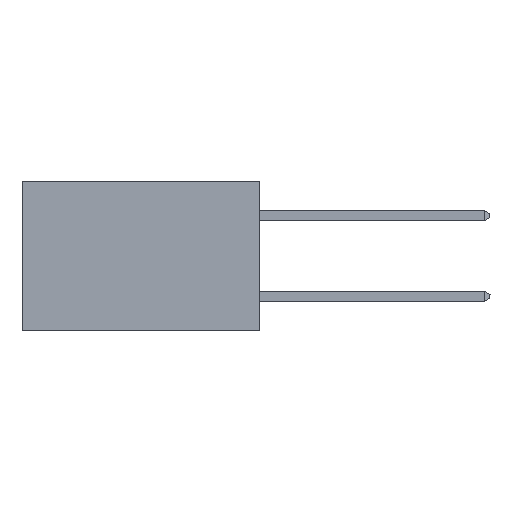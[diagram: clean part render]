
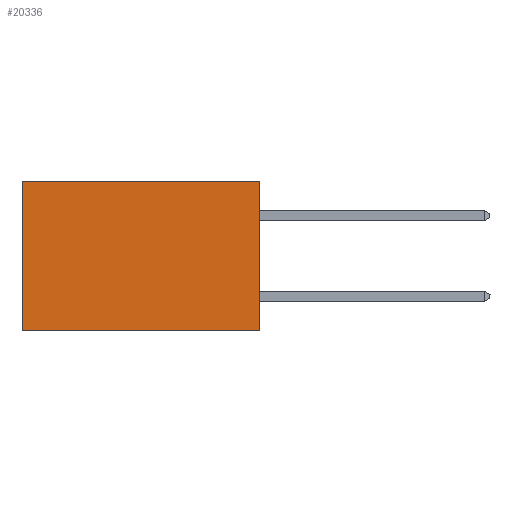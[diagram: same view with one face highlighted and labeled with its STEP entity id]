
A CAD part, left-side view. The second image highlights one B-rep face of the part: STEP entity #20336.
In plain terms, the highlighted planar face has unit normal (-1, 0, 0).
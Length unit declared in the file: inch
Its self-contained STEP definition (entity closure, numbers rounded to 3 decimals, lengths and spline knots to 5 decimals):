
#461 = EDGE_CURVE ( 'NONE', #18956, #10644, #19218, .T. ) ;
#545 = DIRECTION ( 'NONE',  ( 0., 0., -1. ) ) ;
#580 = DIRECTION ( 'NONE',  ( 1., 0., 0. ) ) ;
#1743 = LINE ( 'NONE', #22442, #12050 ) ;
#1756 = VECTOR ( 'NONE', #7344, 39.37008 ) ;
#2547 = VERTEX_POINT ( 'NONE', #8036 ) ;
#5369 = EDGE_CURVE ( 'NONE', #18956, #13268, #1743, .T. ) ;
#6564 = ORIENTED_EDGE ( 'NONE', *, *, #5369, .F. ) ;
#6973 = AXIS2_PLACEMENT_3D ( 'NONE', #13722, #580, #15919 ) ;
#7344 = DIRECTION ( 'NONE',  ( 0., 1., 0. ) ) ;
#7454 = ORIENTED_EDGE ( 'NONE', *, *, #461, .T. ) ;
#8036 = CARTESIAN_POINT ( 'NONE',  ( 0.277, 0.59, -0.37 ) ) ;
#8214 = CARTESIAN_POINT ( 'NONE',  ( 0.277, 0., 0. ) ) ;
#8300 = EDGE_CURVE ( 'NONE', #13268, #2547, #20631, .T. ) ;
#8310 = CARTESIAN_POINT ( 'NONE',  ( 0.277, 0., -0.37 ) ) ;
#8985 = VECTOR ( 'NONE', #18980, 39.37008 ) ;
#10268 = CARTESIAN_POINT ( 'NONE',  ( 0.277, 0., -0.37 ) ) ;
#10487 = VECTOR ( 'NONE', #11620, 39.37008 ) ;
#10644 = VERTEX_POINT ( 'NONE', #19669 ) ;
#10675 = EDGE_LOOP ( 'NONE', ( #12806, #13046, #6564, #7454 ) ) ;
#11620 = DIRECTION ( 'NONE',  ( 0., 0., -1. ) ) ;
#12050 = VECTOR ( 'NONE', #545, 39.37008 ) ;
#12806 = ORIENTED_EDGE ( 'NONE', *, *, #12904, .T. ) ;
#12904 = EDGE_CURVE ( 'NONE', #10644, #2547, #27830, .T. ) ;
#13046 = ORIENTED_EDGE ( 'NONE', *, *, #8300, .F. ) ;
#13268 = VERTEX_POINT ( 'NONE', #8310 ) ;
#13722 = CARTESIAN_POINT ( 'NONE',  ( 0.277, 0., -0.37 ) ) ;
#15919 = DIRECTION ( 'NONE',  ( 0., 0., -1. ) ) ;
#15935 = CARTESIAN_POINT ( 'NONE',  ( 0.277, 0.59, -0.37 ) ) ;
#18956 = VERTEX_POINT ( 'NONE', #22541 ) ;
#18980 = DIRECTION ( 'NONE',  ( 0., 1., 0. ) ) ;
#19218 = LINE ( 'NONE', #8214, #1756 ) ;
#19669 = CARTESIAN_POINT ( 'NONE',  ( 0.277, 0.59, 0. ) ) ;
#20336 = ADVANCED_FACE ( 'NONE', ( #27462 ), #22381, .F. ) ;
#20631 = LINE ( 'NONE', #10268, #8985 ) ;
#22381 = PLANE ( 'NONE',  #6973 ) ;
#22442 = CARTESIAN_POINT ( 'NONE',  ( 0.277, 0., -0.37 ) ) ;
#22541 = CARTESIAN_POINT ( 'NONE',  ( 0.277, 0., 0. ) ) ;
#27462 = FACE_OUTER_BOUND ( 'NONE', #10675, .T. ) ;
#27830 = LINE ( 'NONE', #15935, #10487 ) ;
